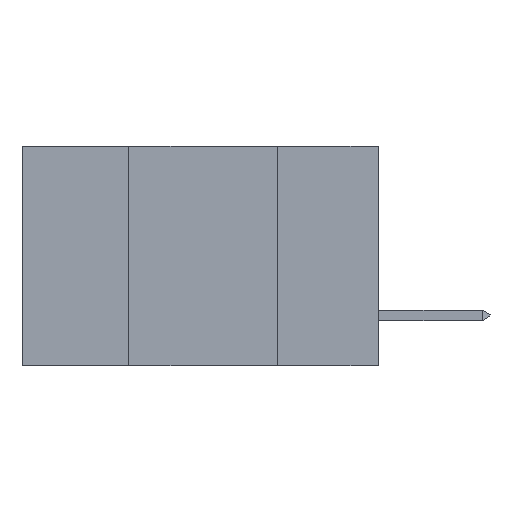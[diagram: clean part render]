
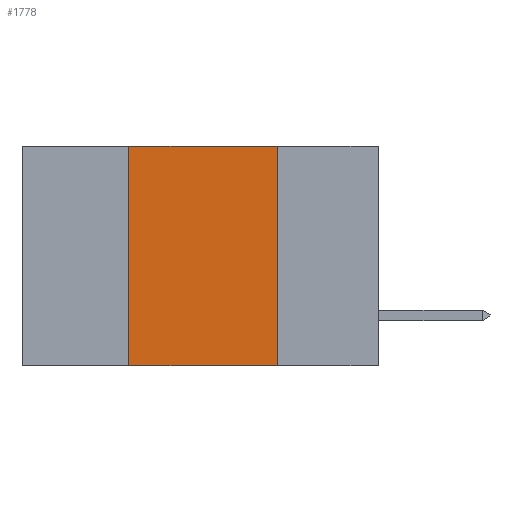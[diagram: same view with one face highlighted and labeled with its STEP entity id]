
A CAD part, left-side view. The second image highlights one B-rep face of the part: STEP entity #1778.
In plain terms, the highlighted planar face has unit normal (-1, 0, 0).
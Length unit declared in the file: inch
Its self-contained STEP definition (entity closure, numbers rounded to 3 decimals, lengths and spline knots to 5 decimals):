
#12 = AXIS2_PLACEMENT_3D ( 'NONE', #10684, #15346, #12175 ) ;
#67 = PLANE ( 'NONE',  #12 ) ;
#844 = VECTOR ( 'NONE', #6484, 39.37008 ) ;
#1419 = EDGE_CURVE ( 'NONE', #3776, #4588, #18043, .T. ) ;
#1778 = ADVANCED_FACE ( 'NONE', ( #16595 ), #67, .F. ) ;
#1925 = VECTOR ( 'NONE', #6744, 39.37008 ) ;
#3211 = CARTESIAN_POINT ( 'NONE',  ( 0., 0.42, 0. ) ) ;
#3632 = CARTESIAN_POINT ( 'NONE',  ( 0., 0.17, -0.37 ) ) ;
#3776 = VERTEX_POINT ( 'NONE', #3211 ) ;
#4185 = DIRECTION ( 'NONE',  ( 0., 0., 1. ) ) ;
#4255 = CARTESIAN_POINT ( 'NONE',  ( 0., 0.17, 0. ) ) ;
#4588 = VERTEX_POINT ( 'NONE', #4255 ) ;
#4970 = EDGE_CURVE ( 'NONE', #4588, #18394, #12852, .T. ) ;
#5703 = CARTESIAN_POINT ( 'NONE',  ( 0., 0.42, -0.37 ) ) ;
#5985 = LINE ( 'NONE', #15886, #1925 ) ;
#6207 = EDGE_CURVE ( 'NONE', #18009, #3776, #7073, .T. ) ;
#6308 = ORIENTED_EDGE ( 'NONE', *, *, #9221, .T. ) ;
#6484 = DIRECTION ( 'NONE',  ( 0., -1., 0. ) ) ;
#6744 = DIRECTION ( 'NONE',  ( 0., -1., 0. ) ) ;
#6760 = ORIENTED_EDGE ( 'NONE', *, *, #4970, .F. ) ;
#6865 = VECTOR ( 'NONE', #8639, 39.37008 ) ;
#7073 = LINE ( 'NONE', #10296, #16361 ) ;
#7899 = EDGE_LOOP ( 'NONE', ( #6760, #15201, #13707, #6308 ) ) ;
#8639 = DIRECTION ( 'NONE',  ( 0., 0., -1. ) ) ;
#9221 = EDGE_CURVE ( 'NONE', #18009, #18394, #5985, .T. ) ;
#10296 = CARTESIAN_POINT ( 'NONE',  ( 0., 0.42, 0. ) ) ;
#10684 = CARTESIAN_POINT ( 'NONE',  ( 0., 0.6, 0. ) ) ;
#11600 = CARTESIAN_POINT ( 'NONE',  ( 0., 0.17, 0. ) ) ;
#12175 = DIRECTION ( 'NONE',  ( 0., 0., -1. ) ) ;
#12852 = LINE ( 'NONE', #11600, #6865 ) ;
#13707 = ORIENTED_EDGE ( 'NONE', *, *, #6207, .F. ) ;
#15201 = ORIENTED_EDGE ( 'NONE', *, *, #1419, .F. ) ;
#15346 = DIRECTION ( 'NONE',  ( 1., 0., 0. ) ) ;
#15622 = CARTESIAN_POINT ( 'NONE',  ( 0., 0.6, 0. ) ) ;
#15886 = CARTESIAN_POINT ( 'NONE',  ( 0., 0.6, -0.37 ) ) ;
#16361 = VECTOR ( 'NONE', #4185, 39.37008 ) ;
#16595 = FACE_OUTER_BOUND ( 'NONE', #7899, .T. ) ;
#18009 = VERTEX_POINT ( 'NONE', #5703 ) ;
#18043 = LINE ( 'NONE', #15622, #844 ) ;
#18394 = VERTEX_POINT ( 'NONE', #3632 ) ;
